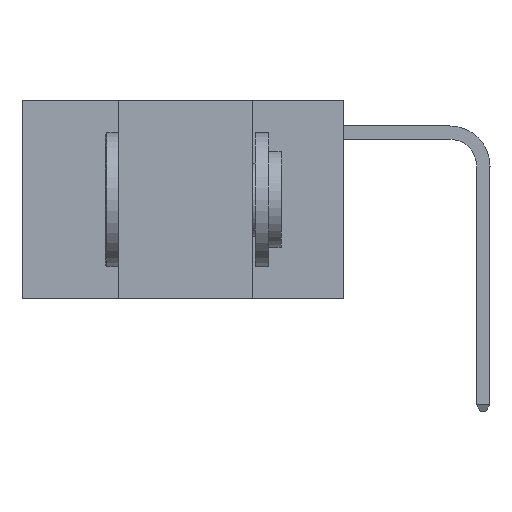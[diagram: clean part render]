
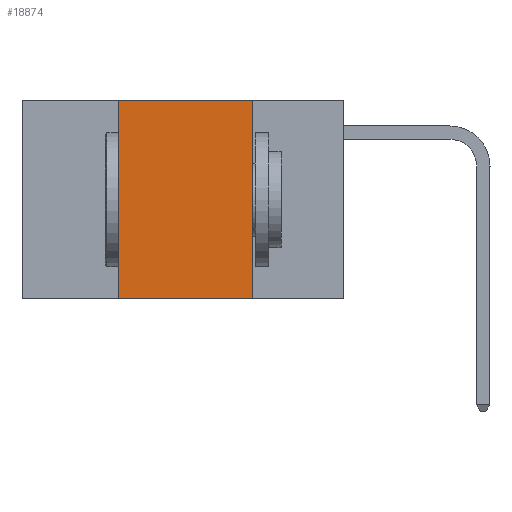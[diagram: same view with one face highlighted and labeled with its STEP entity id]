
A CAD part, left-side view. The second image highlights one B-rep face of the part: STEP entity #18874.
In plain terms, the highlighted planar face has unit normal (-1, 0, 0).
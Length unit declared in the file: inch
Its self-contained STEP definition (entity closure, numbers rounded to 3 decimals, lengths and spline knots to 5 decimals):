
#757 = EDGE_CURVE ( 'NONE', #23702, #17957, #18025, .T. ) ;
#2205 = VECTOR ( 'NONE', #16318, 39.37008 ) ;
#4169 = DIRECTION ( 'NONE',  ( 0., -1., 0. ) ) ;
#5039 = CARTESIAN_POINT ( 'NONE',  ( 0., 0.6, -0.37 ) ) ;
#6819 = VECTOR ( 'NONE', #17780, 39.37008 ) ;
#7394 = DIRECTION ( 'NONE',  ( 0., -1., 0. ) ) ;
#9359 = PLANE ( 'NONE',  #24275 ) ;
#9561 = CARTESIAN_POINT ( 'NONE',  ( 0., 0.42, 0. ) ) ;
#11708 = ORIENTED_EDGE ( 'NONE', *, *, #14124, .T. ) ;
#11799 = VECTOR ( 'NONE', #4169, 39.37008 ) ;
#11864 = CARTESIAN_POINT ( 'NONE',  ( 0., 0.6, 0. ) ) ;
#12774 = VECTOR ( 'NONE', #7394, 39.37008 ) ;
#14053 = CARTESIAN_POINT ( 'NONE',  ( 0., 0.6, 0. ) ) ;
#14124 = EDGE_CURVE ( 'NONE', #25704, #24719, #25231, .T. ) ;
#15334 = CARTESIAN_POINT ( 'NONE',  ( 0., 0.17, -0.37 ) ) ;
#15697 = EDGE_CURVE ( 'NONE', #25704, #23702, #25495, .T. ) ;
#16318 = DIRECTION ( 'NONE',  ( 0., 0., -1. ) ) ;
#16413 = DIRECTION ( 'NONE',  ( 0., 0., -1. ) ) ;
#17780 = DIRECTION ( 'NONE',  ( 0., 0., 1. ) ) ;
#17957 = VERTEX_POINT ( 'NONE', #20165 ) ;
#18025 = LINE ( 'NONE', #11864, #11799 ) ;
#18845 = EDGE_CURVE ( 'NONE', #17957, #24719, #26378, .T. ) ;
#18874 = ADVANCED_FACE ( 'NONE', ( #19444 ), #9359, .F. ) ;
#19444 = FACE_OUTER_BOUND ( 'NONE', #27226, .T. ) ;
#19829 = DIRECTION ( 'NONE',  ( 1., 0., 0. ) ) ;
#20165 = CARTESIAN_POINT ( 'NONE',  ( 0., 0.17, 0. ) ) ;
#22454 = CARTESIAN_POINT ( 'NONE',  ( 0., 0.42, -0.37 ) ) ;
#23702 = VERTEX_POINT ( 'NONE', #9561 ) ;
#23768 = ORIENTED_EDGE ( 'NONE', *, *, #15697, .F. ) ;
#23793 = ORIENTED_EDGE ( 'NONE', *, *, #18845, .F. ) ;
#24275 = AXIS2_PLACEMENT_3D ( 'NONE', #14053, #19829, #16413 ) ;
#24719 = VERTEX_POINT ( 'NONE', #15334 ) ;
#25231 = LINE ( 'NONE', #5039, #12774 ) ;
#25495 = LINE ( 'NONE', #29391, #6819 ) ;
#25704 = VERTEX_POINT ( 'NONE', #22454 ) ;
#26378 = LINE ( 'NONE', #30280, #2205 ) ;
#27226 = EDGE_LOOP ( 'NONE', ( #23793, #30143, #23768, #11708 ) ) ;
#29391 = CARTESIAN_POINT ( 'NONE',  ( 0., 0.42, 0. ) ) ;
#30143 = ORIENTED_EDGE ( 'NONE', *, *, #757, .F. ) ;
#30280 = CARTESIAN_POINT ( 'NONE',  ( 0., 0.17, 0. ) ) ;
